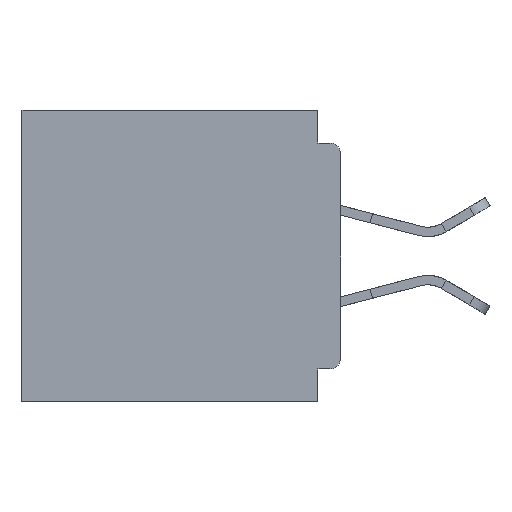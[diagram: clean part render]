
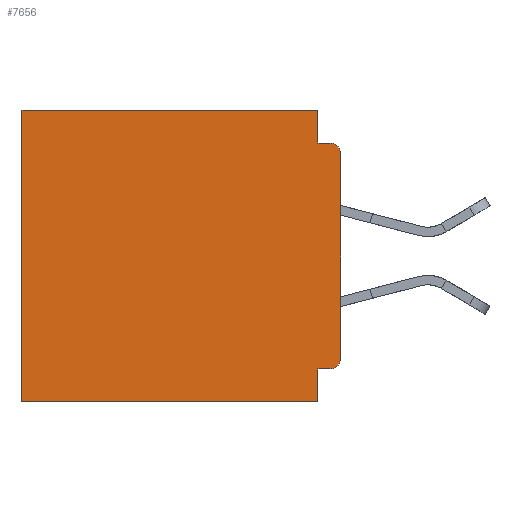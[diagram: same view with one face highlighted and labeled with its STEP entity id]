
A CAD part, left-side view. The second image highlights one B-rep face of the part: STEP entity #7656.
In plain terms, the highlighted planar face has unit normal (-1, 0, 0).
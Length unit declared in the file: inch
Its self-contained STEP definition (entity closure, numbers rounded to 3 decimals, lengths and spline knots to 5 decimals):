
#370 = LINE ( 'NONE', #31480, #39497 ) ;
#419 = CARTESIAN_POINT ( 'NONE',  ( 0.3, 0.031, -0.4 ) ) ;
#515 = ORIENTED_EDGE ( 'NONE', *, *, #42324, .F. ) ;
#840 = DIRECTION ( 'NONE',  ( 0., 1., 0. ) ) ;
#1463 = EDGE_CURVE ( 'NONE', #6190, #42844, #46876, .T. ) ;
#1529 = ORIENTED_EDGE ( 'NONE', *, *, #39863, .T. ) ;
#1999 = VECTOR ( 'NONE', #840, 39.37008 ) ;
#2333 = DIRECTION ( 'NONE',  ( 0., 0., -1. ) ) ;
#3447 = VERTEX_POINT ( 'NONE', #16210 ) ;
#3836 = EDGE_CURVE ( 'NONE', #14819, #34724, #46050, .T. ) ;
#5914 = LINE ( 'NONE', #29684, #16047 ) ;
#6105 = CARTESIAN_POINT ( 'NONE',  ( 0.3, 0., -0.06 ) ) ;
#6190 = VERTEX_POINT ( 'NONE', #37412 ) ;
#6255 = AXIS2_PLACEMENT_3D ( 'NONE', #31722, #9026, #35481 ) ;
#7656 = ADVANCED_FACE ( 'NONE', ( #16892 ), #32615, .F. ) ;
#8701 = DIRECTION ( 'NONE',  ( 0., -1., 0. ) ) ;
#9026 = DIRECTION ( 'NONE',  ( -1., 0., 0. ) ) ;
#9563 = VECTOR ( 'NONE', #8701, 39.37008 ) ;
#11602 = VERTEX_POINT ( 'NONE', #35047 ) ;
#13029 = CARTESIAN_POINT ( 'NONE',  ( 0.3, 0.031, -0.4 ) ) ;
#13658 = LINE ( 'NONE', #17146, #34925 ) ;
#13783 = DIRECTION ( 'NONE',  ( 0., 0., -1. ) ) ;
#13952 = EDGE_CURVE ( 'NONE', #11602, #6190, #13658, .T. ) ;
#14797 = CARTESIAN_POINT ( 'NONE',  ( 0.3, 0.015, -0.355 ) ) ;
#14819 = VERTEX_POINT ( 'NONE', #18230 ) ;
#16047 = VECTOR ( 'NONE', #22095, 39.37008 ) ;
#16210 = CARTESIAN_POINT ( 'NONE',  ( 0.3, 0., -0.34 ) ) ;
#16275 = EDGE_CURVE ( 'NONE', #28578, #3447, #38819, .T. ) ;
#16472 = DIRECTION ( 'NONE',  ( 0., 1., 0. ) ) ;
#16892 = FACE_OUTER_BOUND ( 'NONE', #21600, .T. ) ;
#16927 = DIRECTION ( 'NONE',  ( -1., 0., 0. ) ) ;
#17146 = CARTESIAN_POINT ( 'NONE',  ( 0.3, 0., 0. ) ) ;
#17255 = ORIENTED_EDGE ( 'NONE', *, *, #13952, .T. ) ;
#17689 = ORIENTED_EDGE ( 'NONE', *, *, #16275, .T. ) ;
#18115 = VECTOR ( 'NONE', #23273, 39.37008 ) ;
#18230 = CARTESIAN_POINT ( 'NONE',  ( 0.3, 0.031, -0.045 ) ) ;
#19681 = VERTEX_POINT ( 'NONE', #6105 ) ;
#21281 = CARTESIAN_POINT ( 'NONE',  ( 0.3, 0., -0.4 ) ) ;
#21600 = EDGE_LOOP ( 'NONE', ( #39457, #1529, #26157, #42923, #17255, #44110, #29664, #26594, #515, #17689 ) ) ;
#22095 = DIRECTION ( 'NONE',  ( 0., 0., -1. ) ) ;
#22648 = CARTESIAN_POINT ( 'NONE',  ( 0.3, 0.015, -0.045 ) ) ;
#23273 = DIRECTION ( 'NONE',  ( 0., 0., -1. ) ) ;
#24649 = VECTOR ( 'NONE', #2333, 39.37008 ) ;
#26157 = ORIENTED_EDGE ( 'NONE', *, *, #3836, .F. ) ;
#26594 = ORIENTED_EDGE ( 'NONE', *, *, #44093, .F. ) ;
#27230 = CARTESIAN_POINT ( 'NONE',  ( 0.3, 0., -0.045 ) ) ;
#28168 = LINE ( 'NONE', #419, #18115 ) ;
#28578 = VERTEX_POINT ( 'NONE', #14797 ) ;
#29598 = CARTESIAN_POINT ( 'NONE',  ( 0.3, 0.031, -0.355 ) ) ;
#29664 = ORIENTED_EDGE ( 'NONE', *, *, #30617, .F. ) ;
#29684 = CARTESIAN_POINT ( 'NONE',  ( 0.3, 0.031, 0. ) ) ;
#30617 = EDGE_CURVE ( 'NONE', #43062, #42844, #32273, .T. ) ;
#30771 = CARTESIAN_POINT ( 'NONE',  ( 0.3, 0.437, -0.4 ) ) ;
#31480 = CARTESIAN_POINT ( 'NONE',  ( 0.3, 0., -0.355 ) ) ;
#31722 = CARTESIAN_POINT ( 'NONE',  ( 0.3, 0.015, -0.06 ) ) ;
#32136 = AXIS2_PLACEMENT_3D ( 'NONE', #39464, #16927, #43174 ) ;
#32273 = LINE ( 'NONE', #38636, #1999 ) ;
#32615 = PLANE ( 'NONE',  #38287 ) ;
#33971 = DIRECTION ( 'NONE',  ( 0., 0., -1. ) ) ;
#34599 = LINE ( 'NONE', #40086, #24649 ) ;
#34724 = VERTEX_POINT ( 'NONE', #22648 ) ;
#34925 = VECTOR ( 'NONE', #43418, 39.37008 ) ;
#35047 = CARTESIAN_POINT ( 'NONE',  ( 0.3, 0.031, 0. ) ) ;
#35481 = DIRECTION ( 'NONE',  ( 0., 0., -1. ) ) ;
#36405 = DIRECTION ( 'NONE',  ( 1., 0., 0. ) ) ;
#37412 = CARTESIAN_POINT ( 'NONE',  ( 0.3, 0.437, 0. ) ) ;
#38287 = AXIS2_PLACEMENT_3D ( 'NONE', #21281, #36405, #13783 ) ;
#38636 = CARTESIAN_POINT ( 'NONE',  ( 0.3, 0., -0.4 ) ) ;
#38819 = CIRCLE ( 'NONE', #32136, 0.015 ) ;
#39457 = ORIENTED_EDGE ( 'NONE', *, *, #40012, .F. ) ;
#39464 = CARTESIAN_POINT ( 'NONE',  ( 0.3, 0.015, -0.34 ) ) ;
#39497 = VECTOR ( 'NONE', #16472, 39.37008 ) ;
#39863 = EDGE_CURVE ( 'NONE', #19681, #34724, #41659, .T. ) ;
#40012 = EDGE_CURVE ( 'NONE', #19681, #3447, #34599, .T. ) ;
#40086 = CARTESIAN_POINT ( 'NONE',  ( 0.3, 0., -0.4 ) ) ;
#41659 = CIRCLE ( 'NONE', #6255, 0.015 ) ;
#42324 = EDGE_CURVE ( 'NONE', #28578, #43271, #370, .T. ) ;
#42844 = VERTEX_POINT ( 'NONE', #30771 ) ;
#42923 = ORIENTED_EDGE ( 'NONE', *, *, #46520, .F. ) ;
#43061 = CARTESIAN_POINT ( 'NONE',  ( 0.3, 0.437, -0.4 ) ) ;
#43062 = VERTEX_POINT ( 'NONE', #13029 ) ;
#43174 = DIRECTION ( 'NONE',  ( 0., 0., -1. ) ) ;
#43271 = VERTEX_POINT ( 'NONE', #29598 ) ;
#43418 = DIRECTION ( 'NONE',  ( 0., 1., 0. ) ) ;
#43428 = VECTOR ( 'NONE', #33971, 39.37008 ) ;
#44093 = EDGE_CURVE ( 'NONE', #43271, #43062, #28168, .T. ) ;
#44110 = ORIENTED_EDGE ( 'NONE', *, *, #1463, .T. ) ;
#46050 = LINE ( 'NONE', #27230, #9563 ) ;
#46520 = EDGE_CURVE ( 'NONE', #11602, #14819, #5914, .T. ) ;
#46876 = LINE ( 'NONE', #43061, #43428 ) ;
